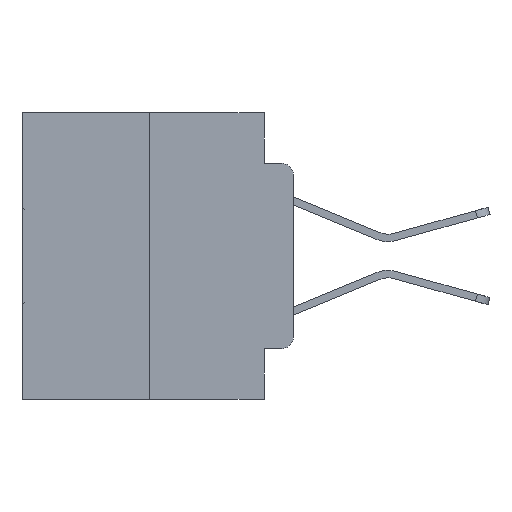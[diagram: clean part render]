
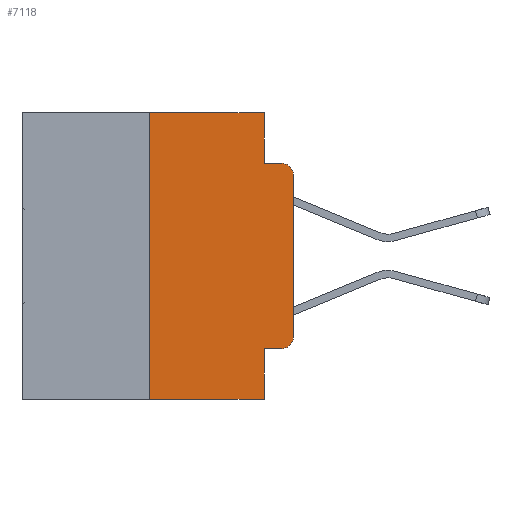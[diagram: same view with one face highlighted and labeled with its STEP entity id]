
A CAD part, left-side view. The second image highlights one B-rep face of the part: STEP entity #7118.
In plain terms, the highlighted planar face has unit normal (-1, 0, 0).
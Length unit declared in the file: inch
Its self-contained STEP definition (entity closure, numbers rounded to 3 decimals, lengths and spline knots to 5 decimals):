
#56 = CARTESIAN_POINT ( 'NONE',  ( 0., 0.473, 0. ) ) ;
#91 = LINE ( 'NONE', #8747, #16915 ) ;
#485 = ORIENTED_EDGE ( 'NONE', *, *, #8420, .T. ) ;
#1113 = EDGE_CURVE ( 'NONE', #1623, #20249, #25244, .T. ) ;
#1235 = DIRECTION ( 'NONE',  ( 0., 0., 1. ) ) ;
#1268 = VERTEX_POINT ( 'NONE', #12754 ) ;
#1623 = VERTEX_POINT ( 'NONE', #26574 ) ;
#2652 = VECTOR ( 'NONE', #18364, 39.37008 ) ;
#3377 = VECTOR ( 'NONE', #9104, 39.37008 ) ;
#3515 = VECTOR ( 'NONE', #6346, 39.37008 ) ;
#4070 = CIRCLE ( 'NONE', #23524, 0.02 ) ;
#4071 = CIRCLE ( 'NONE', #6479, 0.02 ) ;
#4111 = LINE ( 'NONE', #15989, #3377 ) ;
#4456 = CARTESIAN_POINT ( 'NONE',  ( 0., 0.02, -0.3915 ) ) ;
#4560 = VECTOR ( 'NONE', #13887, 39.37008 ) ;
#4785 = EDGE_CURVE ( 'NONE', #1268, #7744, #14996, .T. ) ;
#5179 = ORIENTED_EDGE ( 'NONE', *, *, #23632, .F. ) ;
#5259 = CARTESIAN_POINT ( 'NONE',  ( 0., 0.02, -0.0885 ) ) ;
#5421 = DIRECTION ( 'NONE',  ( -1., 0., 0. ) ) ;
#5658 = EDGE_CURVE ( 'NONE', #1268, #21161, #18507, .T. ) ;
#5833 = VERTEX_POINT ( 'NONE', #18896 ) ;
#6240 = ORIENTED_EDGE ( 'NONE', *, *, #12456, .F. ) ;
#6241 = CARTESIAN_POINT ( 'NONE',  ( 0., 0., -0.1085 ) ) ;
#6312 = EDGE_CURVE ( 'NONE', #16060, #28835, #16698, .T. ) ;
#6346 = DIRECTION ( 'NONE',  ( 0., -1., 0. ) ) ;
#6479 = AXIS2_PLACEMENT_3D ( 'NONE', #4456, #20364, #6742 ) ;
#6742 = DIRECTION ( 'NONE',  ( 0., 0., -1. ) ) ;
#7118 = ADVANCED_FACE ( 'NONE', ( #12751 ), #12178, .F. ) ;
#7744 = VERTEX_POINT ( 'NONE', #8782 ) ;
#8397 = ORIENTED_EDGE ( 'NONE', *, *, #23667, .F. ) ;
#8420 = EDGE_CURVE ( 'NONE', #5833, #1623, #4071, .T. ) ;
#8747 = CARTESIAN_POINT ( 'NONE',  ( 0., 0.051, -0.0885 ) ) ;
#8751 = LINE ( 'NONE', #56, #2652 ) ;
#8782 = CARTESIAN_POINT ( 'NONE',  ( 0., 0.25, 0. ) ) ;
#8797 = VECTOR ( 'NONE', #14136, 39.37008 ) ;
#9104 = DIRECTION ( 'NONE',  ( 0., 0., -1. ) ) ;
#10297 = DIRECTION ( 'NONE',  ( 0., 0., 1. ) ) ;
#11440 = CARTESIAN_POINT ( 'NONE',  ( 0., 0.051, -0.0885 ) ) ;
#11873 = CARTESIAN_POINT ( 'NONE',  ( 0., 0.051, -0.4115 ) ) ;
#12178 = PLANE ( 'NONE',  #19983 ) ;
#12456 = EDGE_CURVE ( 'NONE', #28835, #19935, #91, .T. ) ;
#12695 = ORIENTED_EDGE ( 'NONE', *, *, #29016, .T. ) ;
#12751 = FACE_OUTER_BOUND ( 'NONE', #13652, .T. ) ;
#12754 = CARTESIAN_POINT ( 'NONE',  ( 0., 0.25, -0.5 ) ) ;
#13004 = VERTEX_POINT ( 'NONE', #26407 ) ;
#13652 = EDGE_LOOP ( 'NONE', ( #29184, #12695, #6240, #19764, #8397, #27109, #16606, #5179, #17321, #485 ) ) ;
#13887 = DIRECTION ( 'NONE',  ( 0., 0., -1. ) ) ;
#14136 = DIRECTION ( 'NONE',  ( 0., -1., 0. ) ) ;
#14443 = DIRECTION ( 'NONE',  ( 0., 0., -1. ) ) ;
#14996 = LINE ( 'NONE', #23857, #26263 ) ;
#15989 = CARTESIAN_POINT ( 'NONE',  ( 0., 0.051, 0. ) ) ;
#16060 = VERTEX_POINT ( 'NONE', #26311 ) ;
#16606 = ORIENTED_EDGE ( 'NONE', *, *, #5658, .T. ) ;
#16698 = LINE ( 'NONE', #18373, #4560 ) ;
#16915 = VECTOR ( 'NONE', #29057, 39.37008 ) ;
#17321 = ORIENTED_EDGE ( 'NONE', *, *, #17589, .T. ) ;
#17589 = EDGE_CURVE ( 'NONE', #13004, #5833, #26811, .T. ) ;
#18364 = DIRECTION ( 'NONE',  ( 0., -1., 0. ) ) ;
#18373 = CARTESIAN_POINT ( 'NONE',  ( 0., 0.051, 0. ) ) ;
#18507 = LINE ( 'NONE', #28943, #3515 ) ;
#18896 = CARTESIAN_POINT ( 'NONE',  ( 0., 0.02, -0.4115 ) ) ;
#19061 = CARTESIAN_POINT ( 'NONE',  ( 0., 0.02, -0.1085 ) ) ;
#19764 = ORIENTED_EDGE ( 'NONE', *, *, #6312, .F. ) ;
#19935 = VERTEX_POINT ( 'NONE', #5259 ) ;
#19983 = AXIS2_PLACEMENT_3D ( 'NONE', #23451, #27880, #14443 ) ;
#20249 = VERTEX_POINT ( 'NONE', #6241 ) ;
#20364 = DIRECTION ( 'NONE',  ( -1., 0., 0. ) ) ;
#21161 = VERTEX_POINT ( 'NONE', #27430 ) ;
#21340 = DIRECTION ( 'NONE',  ( 0., 0., -1. ) ) ;
#23451 = CARTESIAN_POINT ( 'NONE',  ( 0., 0.473, 0. ) ) ;
#23524 = AXIS2_PLACEMENT_3D ( 'NONE', #19061, #5421, #21340 ) ;
#23632 = EDGE_CURVE ( 'NONE', #13004, #21161, #4111, .T. ) ;
#23667 = EDGE_CURVE ( 'NONE', #7744, #16060, #8751, .T. ) ;
#23835 = VECTOR ( 'NONE', #1235, 39.37008 ) ;
#23857 = CARTESIAN_POINT ( 'NONE',  ( 0., 0.25, 0. ) ) ;
#25244 = LINE ( 'NONE', #27946, #23835 ) ;
#26263 = VECTOR ( 'NONE', #10297, 39.37008 ) ;
#26311 = CARTESIAN_POINT ( 'NONE',  ( 0., 0.051, 0. ) ) ;
#26407 = CARTESIAN_POINT ( 'NONE',  ( 0., 0.051, -0.4115 ) ) ;
#26574 = CARTESIAN_POINT ( 'NONE',  ( 0., 0., -0.3915 ) ) ;
#26811 = LINE ( 'NONE', #11873, #8797 ) ;
#27109 = ORIENTED_EDGE ( 'NONE', *, *, #4785, .F. ) ;
#27430 = CARTESIAN_POINT ( 'NONE',  ( 0., 0.051, -0.5 ) ) ;
#27880 = DIRECTION ( 'NONE',  ( 1., 0., 0. ) ) ;
#27946 = CARTESIAN_POINT ( 'NONE',  ( 0., 0., 0. ) ) ;
#28835 = VERTEX_POINT ( 'NONE', #11440 ) ;
#28943 = CARTESIAN_POINT ( 'NONE',  ( 0., 0.473, -0.5 ) ) ;
#29016 = EDGE_CURVE ( 'NONE', #20249, #19935, #4070, .T. ) ;
#29057 = DIRECTION ( 'NONE',  ( 0., -1., 0. ) ) ;
#29184 = ORIENTED_EDGE ( 'NONE', *, *, #1113, .T. ) ;
